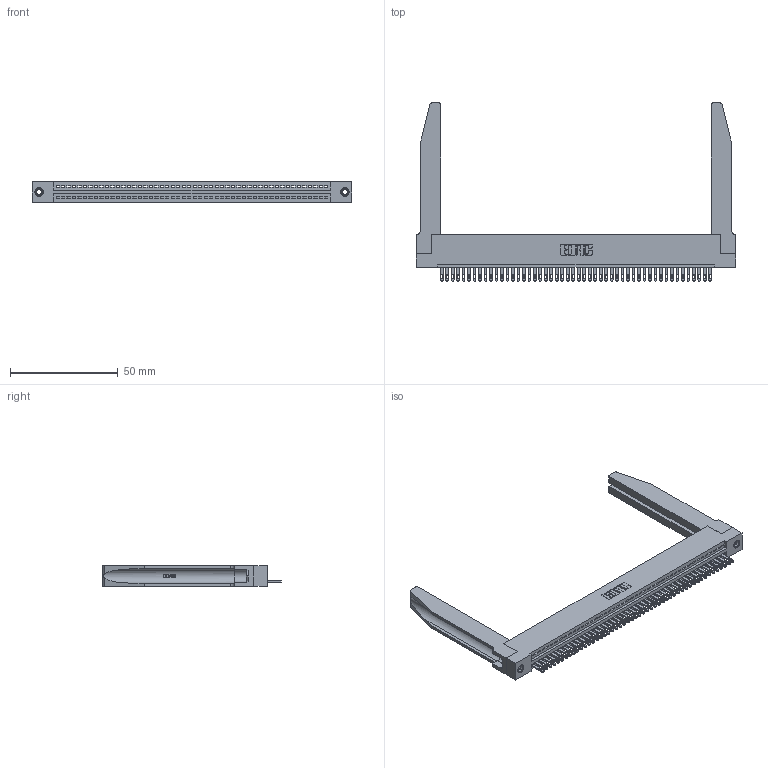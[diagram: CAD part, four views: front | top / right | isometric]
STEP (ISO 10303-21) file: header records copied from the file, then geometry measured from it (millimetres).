
FILE_DESCRIPTION (( 'STEP AP203' ), '1' );
FILE_NAME ('345-050-500-178.STEP', '2019-10-09T10:16:06', ( '' ), ( '' ), 'SwSTEP 2.0', 'SolidWorks 2016', '' );
FILE_SCHEMA (( 'CONFIG_CONTROL_DESIGN' ));
Length unit declared in the file: inch
Products named in the file (5): 345-220-078_345-220-078; 345-250-001_345-250-001-102; 345-050-500-178; 345-292-001_345-293-100; 345 Part_Flush Mounting Lugs - 0.156 Dia-TH
Assembly tree (55 placements, depth 2):
  345-050-500-178
    345 Part_Flush Mounting Lugs - 0.156 Dia-TH
    345-292-001_345-293-100  x50
    345-250-001_345-250-001-102  x2
    345-220-078_345-220-078  x2
Bounding box: 148.23 x 82.47 x 9.4 mm (x, y, z)
Volume: 21946.4 mm3; surface area: 25905.1 mm2
Topology: 55 solids, 55 shells, 3060 faces, 9349 edges, 6222 vertices
Faces by surface type: plane 1922, cylinder 1086, bspline 36, cone 12, torus 4
Entity records: 41224 total; most frequent: CARTESIAN_POINT 8037, ORIENTED_EDGE 6918, DIRECTION 6017, EDGE_CURVE 3459, VECTOR 3029, LINE 3029, VERTEX_POINT 2300, AXIS2_PLACEMENT_3D 1494
